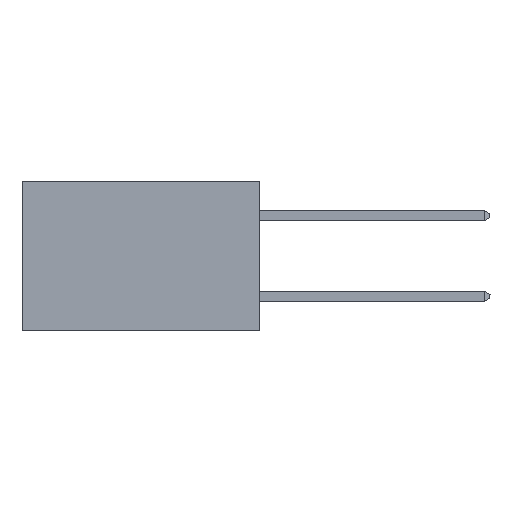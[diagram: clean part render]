
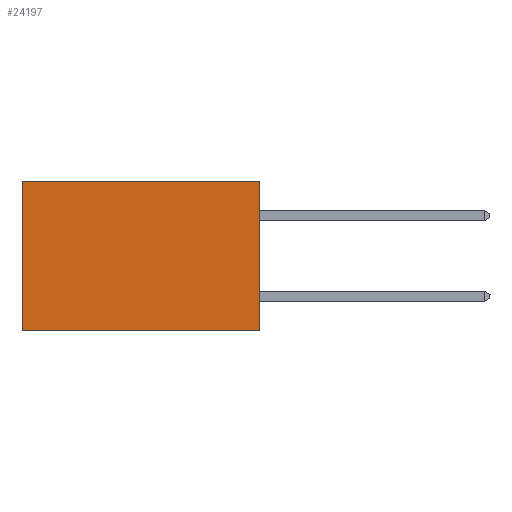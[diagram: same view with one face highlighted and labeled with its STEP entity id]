
A CAD part, left-side view. The second image highlights one B-rep face of the part: STEP entity #24197.
In plain terms, the highlighted planar face has unit normal (-1, 0, 0).
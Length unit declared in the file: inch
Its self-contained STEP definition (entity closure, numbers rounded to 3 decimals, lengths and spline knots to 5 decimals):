
#113 = VECTOR ( 'NONE', #9269, 39.37008 ) ;
#561 = VECTOR ( 'NONE', #28645, 39.37008 ) ;
#893 = DIRECTION ( 'NONE',  ( 0., 1., 0. ) ) ;
#1668 = CARTESIAN_POINT ( 'NONE',  ( 0.277, 0.59, -0.37 ) ) ;
#1763 = EDGE_CURVE ( 'NONE', #30071, #22671, #11383, .T. ) ;
#3718 = VECTOR ( 'NONE', #893, 39.37008 ) ;
#5896 = ORIENTED_EDGE ( 'NONE', *, *, #1763, .T. ) ;
#6075 = AXIS2_PLACEMENT_3D ( 'NONE', #27345, #8920, #25135 ) ;
#6976 = LINE ( 'NONE', #14904, #561 ) ;
#7131 = FACE_OUTER_BOUND ( 'NONE', #29935, .T. ) ;
#7170 = EDGE_CURVE ( 'NONE', #19578, #22671, #27529, .T. ) ;
#8343 = CARTESIAN_POINT ( 'NONE',  ( 0.277, 0.59, -0.37 ) ) ;
#8920 = DIRECTION ( 'NONE',  ( 1., 0., 0. ) ) ;
#8970 = CARTESIAN_POINT ( 'NONE',  ( 0.277, 0.59, 0. ) ) ;
#9065 = VECTOR ( 'NONE', #10356, 39.37008 ) ;
#9269 = DIRECTION ( 'NONE',  ( 0., 0., -1. ) ) ;
#10116 = LINE ( 'NONE', #10481, #3718 ) ;
#10356 = DIRECTION ( 'NONE',  ( 0., 1., 0. ) ) ;
#10481 = CARTESIAN_POINT ( 'NONE',  ( 0.277, 0., 0. ) ) ;
#10649 = CARTESIAN_POINT ( 'NONE',  ( 0.277, 0., -0.37 ) ) ;
#11383 = LINE ( 'NONE', #8343, #113 ) ;
#14468 = ORIENTED_EDGE ( 'NONE', *, *, #24520, .T. ) ;
#14904 = CARTESIAN_POINT ( 'NONE',  ( 0.277, 0., -0.37 ) ) ;
#17837 = CARTESIAN_POINT ( 'NONE',  ( 0.277, 0., -0.37 ) ) ;
#17939 = ORIENTED_EDGE ( 'NONE', *, *, #25858, .F. ) ;
#19578 = VERTEX_POINT ( 'NONE', #17837 ) ;
#22359 = ORIENTED_EDGE ( 'NONE', *, *, #7170, .F. ) ;
#22671 = VERTEX_POINT ( 'NONE', #1668 ) ;
#22840 = PLANE ( 'NONE',  #6075 ) ;
#24197 = ADVANCED_FACE ( 'NONE', ( #7131 ), #22840, .F. ) ;
#24520 = EDGE_CURVE ( 'NONE', #27394, #30071, #10116, .T. ) ;
#25135 = DIRECTION ( 'NONE',  ( 0., 0., -1. ) ) ;
#25858 = EDGE_CURVE ( 'NONE', #27394, #19578, #6976, .T. ) ;
#27345 = CARTESIAN_POINT ( 'NONE',  ( 0.277, 0., -0.37 ) ) ;
#27394 = VERTEX_POINT ( 'NONE', #30084 ) ;
#27529 = LINE ( 'NONE', #10649, #9065 ) ;
#28645 = DIRECTION ( 'NONE',  ( 0., 0., -1. ) ) ;
#29935 = EDGE_LOOP ( 'NONE', ( #5896, #22359, #17939, #14468 ) ) ;
#30071 = VERTEX_POINT ( 'NONE', #8970 ) ;
#30084 = CARTESIAN_POINT ( 'NONE',  ( 0.277, 0., 0. ) ) ;
